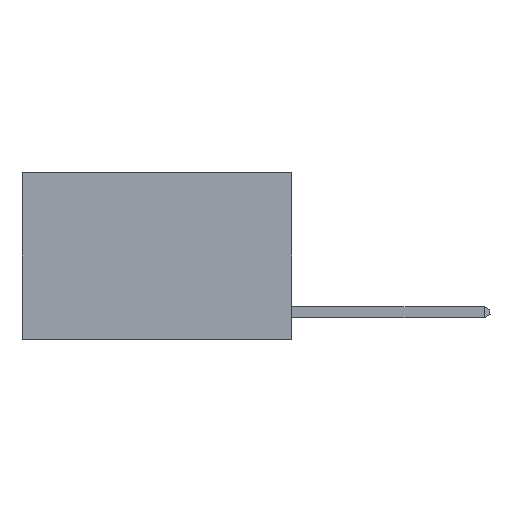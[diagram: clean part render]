
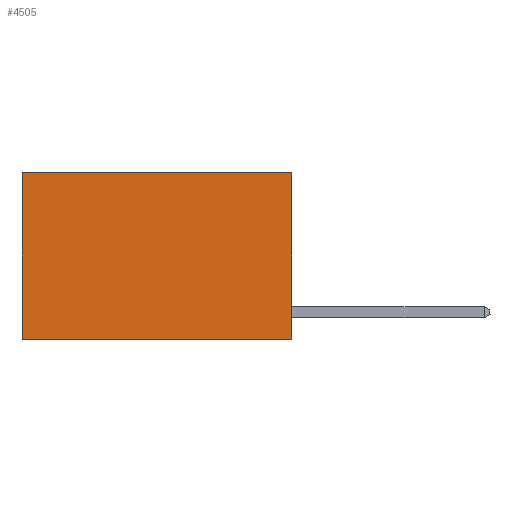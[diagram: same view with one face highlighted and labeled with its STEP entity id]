
A CAD part, left-side view. The second image highlights one B-rep face of the part: STEP entity #4505.
In plain terms, the highlighted planar face has unit normal (-1, 0, 0).
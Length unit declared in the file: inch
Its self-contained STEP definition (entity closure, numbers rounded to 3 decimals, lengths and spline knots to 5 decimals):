
#733 = DIRECTION ( 'NONE',  ( 0., 0., -1. ) ) ;
#1387 = CARTESIAN_POINT ( 'NONE',  ( 0.2625, 0., 0. ) ) ;
#1638 = EDGE_LOOP ( 'NONE', ( #8271, #5753, #16570, #22975 ) ) ;
#2135 = DIRECTION ( 'NONE',  ( 0., 0., -1. ) ) ;
#2738 = VECTOR ( 'NONE', #22198, 39.37008 ) ;
#2847 = CARTESIAN_POINT ( 'NONE',  ( 0.2625, 0.6, 0. ) ) ;
#3882 = CARTESIAN_POINT ( 'NONE',  ( 0.2625, 0., -0.37 ) ) ;
#4240 = CARTESIAN_POINT ( 'NONE',  ( 0.2625, 0., 0. ) ) ;
#4505 = ADVANCED_FACE ( 'NONE', ( #20395 ), #18893, .F. ) ;
#4854 = VECTOR ( 'NONE', #733, 39.37008 ) ;
#5456 = CARTESIAN_POINT ( 'NONE',  ( 0.2625, 0., -0.37 ) ) ;
#5753 = ORIENTED_EDGE ( 'NONE', *, *, #22022, .F. ) ;
#8152 = LINE ( 'NONE', #18900, #9584 ) ;
#8271 = ORIENTED_EDGE ( 'NONE', *, *, #8554, .T. ) ;
#8554 = EDGE_CURVE ( 'NONE', #22848, #9040, #14121, .T. ) ;
#9040 = VERTEX_POINT ( 'NONE', #15364 ) ;
#9584 = VECTOR ( 'NONE', #19780, 39.37008 ) ;
#10973 = EDGE_CURVE ( 'NONE', #13980, #20549, #16164, .T. ) ;
#13980 = VERTEX_POINT ( 'NONE', #1387 ) ;
#14121 = LINE ( 'NONE', #2847, #4854 ) ;
#15364 = CARTESIAN_POINT ( 'NONE',  ( 0.2625, 0.6, -0.37 ) ) ;
#15831 = VECTOR ( 'NONE', #2135, 39.37008 ) ;
#16164 = LINE ( 'NONE', #4240, #15831 ) ;
#16570 = ORIENTED_EDGE ( 'NONE', *, *, #10973, .F. ) ;
#16798 = CARTESIAN_POINT ( 'NONE',  ( 0.2625, 0., 0. ) ) ;
#18400 = CARTESIAN_POINT ( 'NONE',  ( 0.2625, 0.6, 0. ) ) ;
#18893 = PLANE ( 'NONE',  #19403 ) ;
#18900 = CARTESIAN_POINT ( 'NONE',  ( 0.2625, 0., 0. ) ) ;
#19403 = AXIS2_PLACEMENT_3D ( 'NONE', #16798, #20897, #27775 ) ;
#19780 = DIRECTION ( 'NONE',  ( 0., 1., 0. ) ) ;
#20395 = FACE_OUTER_BOUND ( 'NONE', #1638, .T. ) ;
#20549 = VERTEX_POINT ( 'NONE', #5456 ) ;
#20897 = DIRECTION ( 'NONE',  ( 1., 0., 0. ) ) ;
#22022 = EDGE_CURVE ( 'NONE', #20549, #9040, #24890, .T. ) ;
#22198 = DIRECTION ( 'NONE',  ( 0., 1., 0. ) ) ;
#22848 = VERTEX_POINT ( 'NONE', #18400 ) ;
#22975 = ORIENTED_EDGE ( 'NONE', *, *, #26684, .T. ) ;
#24890 = LINE ( 'NONE', #3882, #2738 ) ;
#26684 = EDGE_CURVE ( 'NONE', #13980, #22848, #8152, .T. ) ;
#27775 = DIRECTION ( 'NONE',  ( 0., 0., -1. ) ) ;
